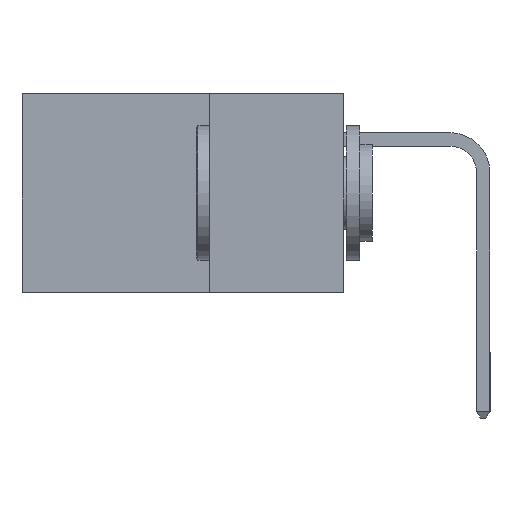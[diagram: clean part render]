
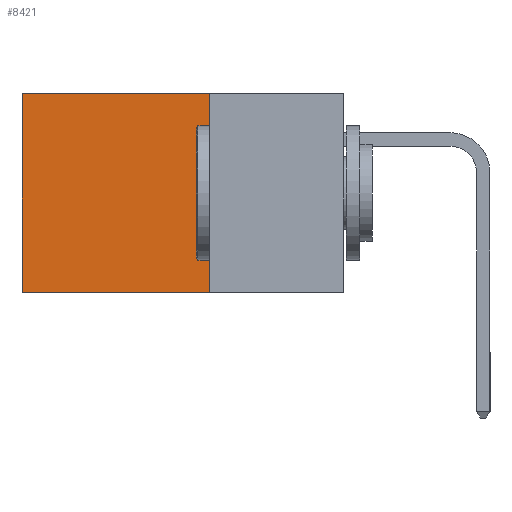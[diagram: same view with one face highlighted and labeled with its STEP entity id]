
A CAD part, left-side view. The second image highlights one B-rep face of the part: STEP entity #8421.
In plain terms, the highlighted planar face has unit normal (-1, 0, 0).
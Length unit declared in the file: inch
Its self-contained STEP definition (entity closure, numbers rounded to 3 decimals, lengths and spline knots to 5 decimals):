
#8 = EDGE_CURVE ( 'NONE', #12197, #8702, #2917, .T. ) ;
#410 = DIRECTION ( 'NONE',  ( 0., 0., -1. ) ) ;
#1029 = CARTESIAN_POINT ( 'NONE',  ( 0.2615, 0.25, 0. ) ) ;
#1246 = ORIENTED_EDGE ( 'NONE', *, *, #2387, .F. ) ;
#1260 = VERTEX_POINT ( 'NONE', #3591 ) ;
#1541 = DIRECTION ( 'NONE',  ( 0., 0., -1. ) ) ;
#1999 = VECTOR ( 'NONE', #1541, 39.37008 ) ;
#2015 = VECTOR ( 'NONE', #12206, 39.37008 ) ;
#2340 = CARTESIAN_POINT ( 'NONE',  ( 0.2615, 0.25, -0.37 ) ) ;
#2387 = EDGE_CURVE ( 'NONE', #12197, #1260, #12769, .T. ) ;
#2582 = EDGE_CURVE ( 'NONE', #1260, #9975, #3925, .T. ) ;
#2889 = CARTESIAN_POINT ( 'NONE',  ( 0.2615, 0.6, -0.37 ) ) ;
#2917 = LINE ( 'NONE', #1029, #7378 ) ;
#3132 = ORIENTED_EDGE ( 'NONE', *, *, #12175, .T. ) ;
#3591 = CARTESIAN_POINT ( 'NONE',  ( 0.2615, 0.25, -0.37 ) ) ;
#3925 = LINE ( 'NONE', #12277, #2015 ) ;
#4073 = AXIS2_PLACEMENT_3D ( 'NONE', #2340, #6729, #4565 ) ;
#4505 = PLANE ( 'NONE',  #4073 ) ;
#4565 = DIRECTION ( 'NONE',  ( 0., 0., -1. ) ) ;
#5535 = EDGE_LOOP ( 'NONE', ( #3132, #7821, #1246, #11353 ) ) ;
#5950 = CARTESIAN_POINT ( 'NONE',  ( 0.2615, 0.6, -0.37 ) ) ;
#5973 = DIRECTION ( 'NONE',  ( 0., 1., 0. ) ) ;
#6729 = DIRECTION ( 'NONE',  ( 1., 0., 0. ) ) ;
#7378 = VECTOR ( 'NONE', #5973, 39.37008 ) ;
#7579 = CARTESIAN_POINT ( 'NONE',  ( 0.2615, 0.25, -0.37 ) ) ;
#7616 = FACE_OUTER_BOUND ( 'NONE', #5535, .T. ) ;
#7821 = ORIENTED_EDGE ( 'NONE', *, *, #2582, .F. ) ;
#8421 = ADVANCED_FACE ( 'NONE', ( #7616 ), #4505, .F. ) ;
#8702 = VERTEX_POINT ( 'NONE', #11268 ) ;
#9975 = VERTEX_POINT ( 'NONE', #2889 ) ;
#11268 = CARTESIAN_POINT ( 'NONE',  ( 0.2615, 0.6, 0. ) ) ;
#11309 = VECTOR ( 'NONE', #410, 39.37008 ) ;
#11353 = ORIENTED_EDGE ( 'NONE', *, *, #8, .T. ) ;
#12175 = EDGE_CURVE ( 'NONE', #8702, #9975, #13092, .T. ) ;
#12197 = VERTEX_POINT ( 'NONE', #13159 ) ;
#12206 = DIRECTION ( 'NONE',  ( 0., 1., 0. ) ) ;
#12277 = CARTESIAN_POINT ( 'NONE',  ( 0.2615, 0.25, -0.37 ) ) ;
#12769 = LINE ( 'NONE', #7579, #11309 ) ;
#13092 = LINE ( 'NONE', #5950, #1999 ) ;
#13159 = CARTESIAN_POINT ( 'NONE',  ( 0.2615, 0.25, 0. ) ) ;
